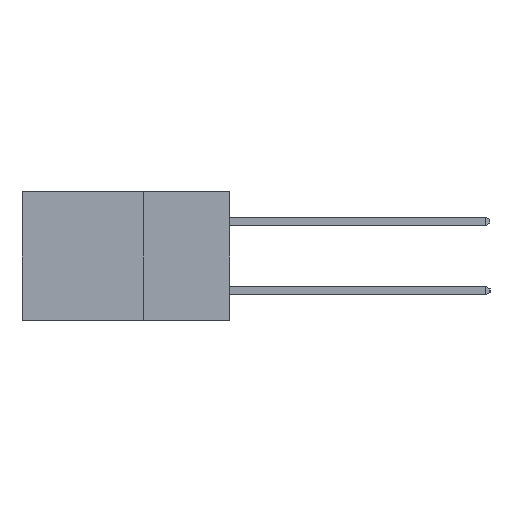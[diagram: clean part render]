
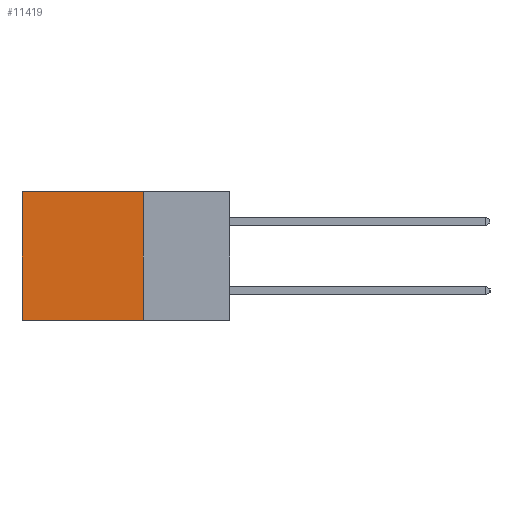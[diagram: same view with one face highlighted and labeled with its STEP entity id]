
A CAD part, left-side view. The second image highlights one B-rep face of the part: STEP entity #11419.
In plain terms, the highlighted planar face has unit normal (-1, 0, 0).
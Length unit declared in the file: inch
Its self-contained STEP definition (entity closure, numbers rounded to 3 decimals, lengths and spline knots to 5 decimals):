
#418 = VERTEX_POINT ( 'NONE', #6658 ) ;
#460 = PLANE ( 'NONE',  #7922 ) ;
#720 = VERTEX_POINT ( 'NONE', #17238 ) ;
#823 = ORIENTED_EDGE ( 'NONE', *, *, #1401, .F. ) ;
#1140 = VECTOR ( 'NONE', #19546, 39.37008 ) ;
#1294 = LINE ( 'NONE', #2596, #17557 ) ;
#1401 = EDGE_CURVE ( 'NONE', #11044, #418, #5557, .T. ) ;
#2466 = VECTOR ( 'NONE', #8414, 39.37008 ) ;
#2596 = CARTESIAN_POINT ( 'NONE',  ( 0.2615, 0.25, -0.37 ) ) ;
#5557 = LINE ( 'NONE', #19616, #1140 ) ;
#6092 = EDGE_LOOP ( 'NONE', ( #7473, #823, #8030, #20376 ) ) ;
#6658 = CARTESIAN_POINT ( 'NONE',  ( 0.2615, 0.6, -0.37 ) ) ;
#6993 = LINE ( 'NONE', #15253, #10289 ) ;
#7473 = ORIENTED_EDGE ( 'NONE', *, *, #12521, .T. ) ;
#7832 = CARTESIAN_POINT ( 'NONE',  ( 0.2615, 0.25, -0.37 ) ) ;
#7922 = AXIS2_PLACEMENT_3D ( 'NONE', #18386, #8729, #20005 ) ;
#8030 = ORIENTED_EDGE ( 'NONE', *, *, #19166, .F. ) ;
#8044 = VERTEX_POINT ( 'NONE', #12421 ) ;
#8414 = DIRECTION ( 'NONE',  ( 0., 1., 0. ) ) ;
#8729 = DIRECTION ( 'NONE',  ( 1., 0., 0. ) ) ;
#10289 = VECTOR ( 'NONE', #16866, 39.37008 ) ;
#11044 = VERTEX_POINT ( 'NONE', #7832 ) ;
#11419 = ADVANCED_FACE ( 'NONE', ( #13853 ), #460, .F. ) ;
#12373 = DIRECTION ( 'NONE',  ( 0., 0., -1. ) ) ;
#12421 = CARTESIAN_POINT ( 'NONE',  ( 0.2615, 0.6, 0. ) ) ;
#12521 = EDGE_CURVE ( 'NONE', #8044, #418, #6993, .T. ) ;
#13853 = FACE_OUTER_BOUND ( 'NONE', #6092, .T. ) ;
#15253 = CARTESIAN_POINT ( 'NONE',  ( 0.2615, 0.6, -0.37 ) ) ;
#15740 = EDGE_CURVE ( 'NONE', #720, #8044, #18703, .T. ) ;
#16866 = DIRECTION ( 'NONE',  ( 0., 0., -1. ) ) ;
#17238 = CARTESIAN_POINT ( 'NONE',  ( 0.2615, 0.25, 0. ) ) ;
#17557 = VECTOR ( 'NONE', #12373, 39.37008 ) ;
#18386 = CARTESIAN_POINT ( 'NONE',  ( 0.2615, 0.25, -0.37 ) ) ;
#18703 = LINE ( 'NONE', #19689, #2466 ) ;
#19166 = EDGE_CURVE ( 'NONE', #720, #11044, #1294, .T. ) ;
#19546 = DIRECTION ( 'NONE',  ( 0., 1., 0. ) ) ;
#19616 = CARTESIAN_POINT ( 'NONE',  ( 0.2615, 0.25, -0.37 ) ) ;
#19689 = CARTESIAN_POINT ( 'NONE',  ( 0.2615, 0.25, 0. ) ) ;
#20005 = DIRECTION ( 'NONE',  ( 0., 0., -1. ) ) ;
#20376 = ORIENTED_EDGE ( 'NONE', *, *, #15740, .T. ) ;
